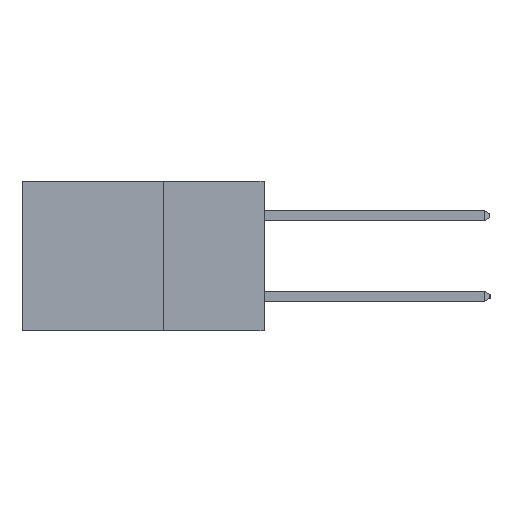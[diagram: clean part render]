
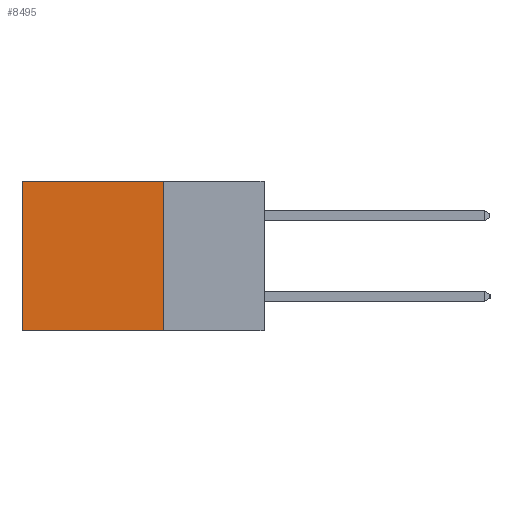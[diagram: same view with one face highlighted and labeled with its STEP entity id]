
A CAD part, left-side view. The second image highlights one B-rep face of the part: STEP entity #8495.
In plain terms, the highlighted planar face has unit normal (-1, 0, 0).
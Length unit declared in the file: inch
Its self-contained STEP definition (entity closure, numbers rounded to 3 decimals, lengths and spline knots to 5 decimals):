
#277 = DIRECTION ( 'NONE',  ( 0., 1., 0. ) ) ;
#470 = CARTESIAN_POINT ( 'NONE',  ( 0.2615, 0.25, -0.37 ) ) ;
#834 = VECTOR ( 'NONE', #6311, 39.37008 ) ;
#1814 = ORIENTED_EDGE ( 'NONE', *, *, #3915, .F. ) ;
#2410 = ORIENTED_EDGE ( 'NONE', *, *, #11282, .F. ) ;
#2778 = EDGE_CURVE ( 'NONE', #7530, #9777, #12446, .T. ) ;
#3215 = CARTESIAN_POINT ( 'NONE',  ( 0.2615, 0.6, -0.37 ) ) ;
#3221 = LINE ( 'NONE', #12500, #9147 ) ;
#3271 = EDGE_LOOP ( 'NONE', ( #7517, #1814, #2410, #3379 ) ) ;
#3379 = ORIENTED_EDGE ( 'NONE', *, *, #2778, .T. ) ;
#3915 = EDGE_CURVE ( 'NONE', #4578, #5374, #10969, .T. ) ;
#4578 = VERTEX_POINT ( 'NONE', #9445 ) ;
#4653 = FACE_OUTER_BOUND ( 'NONE', #3271, .T. ) ;
#5125 = AXIS2_PLACEMENT_3D ( 'NONE', #5518, #5462, #5411 ) ;
#5374 = VERTEX_POINT ( 'NONE', #3215 ) ;
#5411 = DIRECTION ( 'NONE',  ( 0., 0., -1. ) ) ;
#5462 = DIRECTION ( 'NONE',  ( 1., 0., 0. ) ) ;
#5518 = CARTESIAN_POINT ( 'NONE',  ( 0.2615, 0.25, -0.37 ) ) ;
#5600 = PLANE ( 'NONE',  #5125 ) ;
#5605 = DIRECTION ( 'NONE',  ( 0., 0., -1. ) ) ;
#6157 = VECTOR ( 'NONE', #6955, 39.37008 ) ;
#6311 = DIRECTION ( 'NONE',  ( 0., 1., 0. ) ) ;
#6340 = CARTESIAN_POINT ( 'NONE',  ( 0.2615, 0.25, 0. ) ) ;
#6955 = DIRECTION ( 'NONE',  ( 0., 0., -1. ) ) ;
#6990 = CARTESIAN_POINT ( 'NONE',  ( 0.2615, 0.25, -0.37 ) ) ;
#7517 = ORIENTED_EDGE ( 'NONE', *, *, #14037, .T. ) ;
#7530 = VERTEX_POINT ( 'NONE', #14761 ) ;
#7577 = VECTOR ( 'NONE', #277, 39.37008 ) ;
#8495 = ADVANCED_FACE ( 'NONE', ( #4653 ), #5600, .F. ) ;
#9147 = VECTOR ( 'NONE', #5605, 39.37008 ) ;
#9445 = CARTESIAN_POINT ( 'NONE',  ( 0.2615, 0.25, -0.37 ) ) ;
#9777 = VERTEX_POINT ( 'NONE', #12299 ) ;
#10969 = LINE ( 'NONE', #470, #7577 ) ;
#11282 = EDGE_CURVE ( 'NONE', #7530, #4578, #12261, .T. ) ;
#12261 = LINE ( 'NONE', #6990, #6157 ) ;
#12299 = CARTESIAN_POINT ( 'NONE',  ( 0.2615, 0.6, 0. ) ) ;
#12446 = LINE ( 'NONE', #6340, #834 ) ;
#12500 = CARTESIAN_POINT ( 'NONE',  ( 0.2615, 0.6, -0.37 ) ) ;
#14037 = EDGE_CURVE ( 'NONE', #9777, #5374, #3221, .T. ) ;
#14761 = CARTESIAN_POINT ( 'NONE',  ( 0.2615, 0.25, 0. ) ) ;
